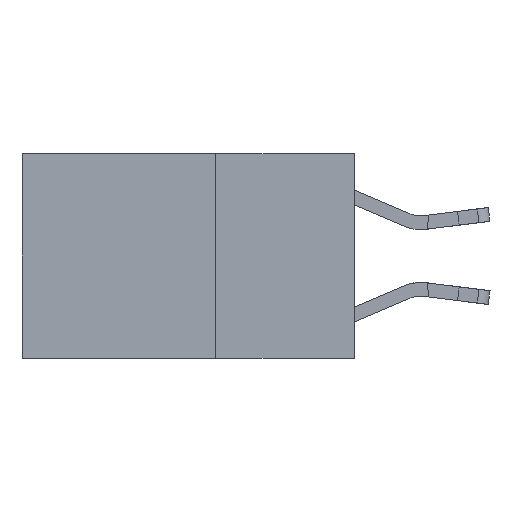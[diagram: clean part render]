
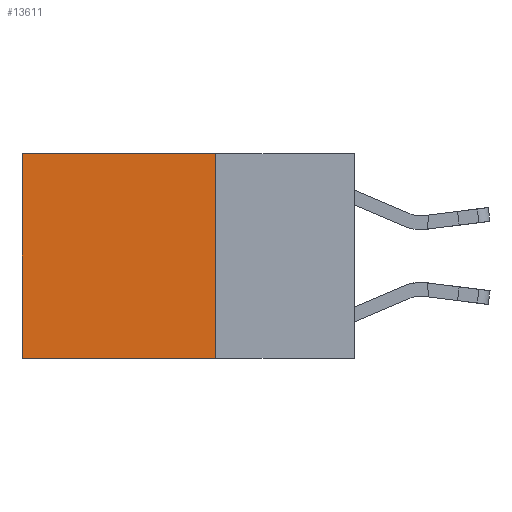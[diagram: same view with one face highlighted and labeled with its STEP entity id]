
A CAD part, left-side view. The second image highlights one B-rep face of the part: STEP entity #13611.
In plain terms, the highlighted planar face has unit normal (-1, 0, 0).
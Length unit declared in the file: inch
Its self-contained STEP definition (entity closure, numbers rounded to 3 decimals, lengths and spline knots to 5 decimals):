
#794 = EDGE_LOOP ( 'NONE', ( #7395, #11920, #6720, #12441 ) ) ;
#1671 = LINE ( 'NONE', #1766, #14528 ) ;
#1766 = CARTESIAN_POINT ( 'NONE',  ( 0.2625, 0.25, -0.37 ) ) ;
#2237 = CARTESIAN_POINT ( 'NONE',  ( 0.2625, 0.6, 0. ) ) ;
#2425 = PLANE ( 'NONE',  #12029 ) ;
#2655 = VERTEX_POINT ( 'NONE', #13743 ) ;
#3266 = EDGE_CURVE ( 'NONE', #10040, #2655, #1671, .T. ) ;
#3666 = DIRECTION ( 'NONE',  ( 0., 0., -1. ) ) ;
#3970 = VECTOR ( 'NONE', #9616, 39.37008 ) ;
#4445 = CARTESIAN_POINT ( 'NONE',  ( 0.2625, 0.25, 0. ) ) ;
#5507 = VECTOR ( 'NONE', #3666, 39.37008 ) ;
#6063 = DIRECTION ( 'NONE',  ( 1., 0., 0. ) ) ;
#6720 = ORIENTED_EDGE ( 'NONE', *, *, #13758, .F. ) ;
#7395 = ORIENTED_EDGE ( 'NONE', *, *, #15935, .T. ) ;
#7572 = VECTOR ( 'NONE', #12338, 39.37008 ) ;
#7715 = CARTESIAN_POINT ( 'NONE',  ( 0.2625, 0.6, 0. ) ) ;
#8226 = LINE ( 'NONE', #7715, #3970 ) ;
#9616 = DIRECTION ( 'NONE',  ( 0., 0., -1. ) ) ;
#10040 = VERTEX_POINT ( 'NONE', #16931 ) ;
#10322 = CARTESIAN_POINT ( 'NONE',  ( 0.2625, 0.25, 0. ) ) ;
#10684 = FACE_OUTER_BOUND ( 'NONE', #794, .T. ) ;
#11914 = LINE ( 'NONE', #15535, #7572 ) ;
#11920 = ORIENTED_EDGE ( 'NONE', *, *, #3266, .F. ) ;
#12029 = AXIS2_PLACEMENT_3D ( 'NONE', #4445, #6063, #14123 ) ;
#12338 = DIRECTION ( 'NONE',  ( 0., 1., 0. ) ) ;
#12441 = ORIENTED_EDGE ( 'NONE', *, *, #14361, .T. ) ;
#12991 = VERTEX_POINT ( 'NONE', #2237 ) ;
#13611 = ADVANCED_FACE ( 'NONE', ( #10684 ), #2425, .F. ) ;
#13743 = CARTESIAN_POINT ( 'NONE',  ( 0.2625, 0.6, -0.37 ) ) ;
#13758 = EDGE_CURVE ( 'NONE', #18843, #10040, #19786, .T. ) ;
#14123 = DIRECTION ( 'NONE',  ( 0., 0., -1. ) ) ;
#14361 = EDGE_CURVE ( 'NONE', #18843, #12991, #11914, .T. ) ;
#14528 = VECTOR ( 'NONE', #14851, 39.37008 ) ;
#14851 = DIRECTION ( 'NONE',  ( 0., 1., 0. ) ) ;
#15535 = CARTESIAN_POINT ( 'NONE',  ( 0.2625, 0.25, 0. ) ) ;
#15935 = EDGE_CURVE ( 'NONE', #12991, #2655, #8226, .T. ) ;
#16931 = CARTESIAN_POINT ( 'NONE',  ( 0.2625, 0.25, -0.37 ) ) ;
#18357 = CARTESIAN_POINT ( 'NONE',  ( 0.2625, 0.25, 0. ) ) ;
#18843 = VERTEX_POINT ( 'NONE', #10322 ) ;
#19786 = LINE ( 'NONE', #18357, #5507 ) ;
